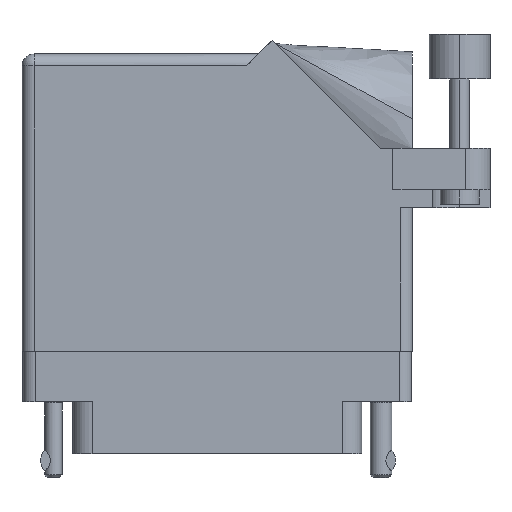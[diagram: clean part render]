
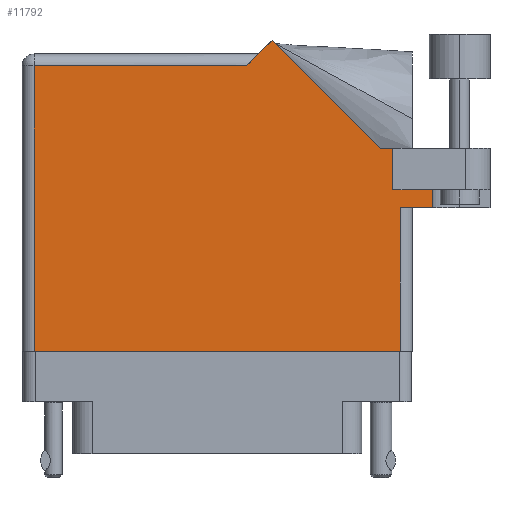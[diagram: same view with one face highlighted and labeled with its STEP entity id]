
A CAD part, front view. The second image highlights one B-rep face of the part: STEP entity #11792.
In plain terms, the highlighted face is planar.
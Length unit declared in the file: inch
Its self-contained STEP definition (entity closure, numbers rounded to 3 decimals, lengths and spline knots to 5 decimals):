
#990 = LINE ( 'NONE', #33582, #6879 ) ;
#1354 = ORIENTED_EDGE ( 'NONE', *, *, #5751, .T. ) ;
#2947 = CARTESIAN_POINT ( 'NONE',  ( 0., 1.53, 0. ) ) ;
#3234 = CARTESIAN_POINT ( 'NONE',  ( 1.91, 0.831, 0. ) ) ;
#4028 = CARTESIAN_POINT ( 'NONE',  ( 1.217, 1.53, 0. ) ) ;
#4146 = CARTESIAN_POINT ( 'NONE',  ( 0., 0., 0. ) ) ;
#4919 = CARTESIAN_POINT ( 'NONE',  ( 1.948, 0., 0. ) ) ;
#5751 = EDGE_CURVE ( 'NONE', #32708, #19872, #19036, .T. ) ;
#5757 = VECTOR ( 'NONE', #34159, 39.37008 ) ;
#6306 = LINE ( 'NONE', #43594, #44927 ) ;
#6641 = CARTESIAN_POINT ( 'NONE',  ( 1.91, 0.831, 0. ) ) ;
#6879 = VECTOR ( 'NONE', #7696, 39.37008 ) ;
#7042 = DIRECTION ( 'NONE',  ( -1., 0., 0. ) ) ;
#7444 = VECTOR ( 'NONE', #9508, 39.37008 ) ;
#7696 = DIRECTION ( 'NONE',  ( 0., -1., 0. ) ) ;
#8265 = FACE_OUTER_BOUND ( 'NONE', #32116, .T. ) ;
#8510 = LINE ( 'NONE', #40022, #17301 ) ;
#9508 = DIRECTION ( 'NONE',  ( -1., 0., 0. ) ) ;
#9732 = DIRECTION ( 'NONE',  ( 0., 1., 0. ) ) ;
#10441 = VERTEX_POINT ( 'NONE', #39763 ) ;
#10484 = EDGE_CURVE ( 'NONE', #25265, #26526, #45860, .T. ) ;
#10530 = CARTESIAN_POINT ( 'NONE',  ( 1.84442, 1.044, 0. ) ) ;
#11084 = ORIENTED_EDGE ( 'NONE', *, *, #30466, .T. ) ;
#11167 = VERTEX_POINT ( 'NONE', #33609 ) ;
#11792 = ADVANCED_FACE ( 'NONE', ( #8265 ), #36676, .F. ) ;
#12435 = VECTOR ( 'NONE', #26130, 39.37008 ) ;
#13024 = EDGE_CURVE ( 'NONE', #11167, #14028, #32784, .T. ) ;
#13460 = CARTESIAN_POINT ( 'NONE',  ( 1.948, 0.737, 0. ) ) ;
#13590 = ORIENTED_EDGE ( 'NONE', *, *, #48249, .T. ) ;
#13799 = VECTOR ( 'NONE', #9732, 39.37008 ) ;
#14028 = VERTEX_POINT ( 'NONE', #37925 ) ;
#14407 = EDGE_CURVE ( 'NONE', #19872, #45333, #6306, .T. ) ;
#14605 = EDGE_CURVE ( 'NONE', #26526, #11167, #41418, .T. ) ;
#16339 = VECTOR ( 'NONE', #47357, 39.37008 ) ;
#17117 = CARTESIAN_POINT ( 'NONE',  ( 2.1115, 0.831, 0. ) ) ;
#17301 = VECTOR ( 'NONE', #39360, 39.37008 ) ;
#18623 = LINE ( 'NONE', #4028, #5757 ) ;
#18814 = ORIENTED_EDGE ( 'NONE', *, *, #29938, .T. ) ;
#19036 = LINE ( 'NONE', #13460, #13799 ) ;
#19609 = CARTESIAN_POINT ( 'NONE',  ( 2.1115, 0.737, 0. ) ) ;
#19872 = VERTEX_POINT ( 'NONE', #42910 ) ;
#20058 = VERTEX_POINT ( 'NONE', #43712 ) ;
#20728 = ORIENTED_EDGE ( 'NONE', *, *, #45939, .F. ) ;
#21000 = ORIENTED_EDGE ( 'NONE', *, *, #13024, .T. ) ;
#21211 = DIRECTION ( 'NONE',  ( 1., 0., 0. ) ) ;
#23358 = ORIENTED_EDGE ( 'NONE', *, *, #14605, .T. ) ;
#25265 = VERTEX_POINT ( 'NONE', #6641 ) ;
#25728 = DIRECTION ( 'NONE',  ( 0., 0., -1. ) ) ;
#26130 = DIRECTION ( 'NONE',  ( 1., 0., 0. ) ) ;
#26526 = VERTEX_POINT ( 'NONE', #42178 ) ;
#26621 = LINE ( 'NONE', #32329, #41251 ) ;
#27088 = EDGE_CURVE ( 'NONE', #41062, #32708, #33568, .T. ) ;
#27171 = ORIENTED_EDGE ( 'NONE', *, *, #10484, .T. ) ;
#28191 = ORIENTED_EDGE ( 'NONE', *, *, #32321, .F. ) ;
#28197 = CARTESIAN_POINT ( 'NONE',  ( 0., 1.468, 0. ) ) ;
#29938 = EDGE_CURVE ( 'NONE', #14028, #10441, #18623, .T. ) ;
#30110 = CARTESIAN_POINT ( 'NONE',  ( 0.062, 0., 0. ) ) ;
#30195 = CARTESIAN_POINT ( 'NONE',  ( 2.41, 1.044, 0. ) ) ;
#30466 = EDGE_CURVE ( 'NONE', #10441, #20058, #34420, .T. ) ;
#30688 = DIRECTION ( 'NONE',  ( -1., 0., 0. ) ) ;
#32116 = EDGE_LOOP ( 'NONE', ( #41362, #1354, #46686, #20728, #28191, #27171, #23358, #21000, #18814, #11084, #13590 ) ) ;
#32321 = EDGE_CURVE ( 'NONE', #25265, #33697, #8510, .T. ) ;
#32329 = CARTESIAN_POINT ( 'NONE',  ( 0.062, 0., 0. ) ) ;
#32708 = VERTEX_POINT ( 'NONE', #4919 ) ;
#32784 = LINE ( 'NONE', #10530, #16339 ) ;
#33568 = LINE ( 'NONE', #4146, #12435 ) ;
#33582 = CARTESIAN_POINT ( 'NONE',  ( 2.1115, 1.16177, 0. ) ) ;
#33609 = CARTESIAN_POINT ( 'NONE',  ( 1.84442, 1.044, 0. ) ) ;
#33697 = VERTEX_POINT ( 'NONE', #17117 ) ;
#34159 = DIRECTION ( 'NONE',  ( -0.707, -0.707, 0. ) ) ;
#34420 = LINE ( 'NONE', #28197, #7444 ) ;
#35593 = DIRECTION ( 'NONE',  ( 0., -1., 0. ) ) ;
#35955 = VECTOR ( 'NONE', #37109, 39.37008 ) ;
#36676 = PLANE ( 'NONE',  #38304 ) ;
#37109 = DIRECTION ( 'NONE',  ( 0., 1., 0. ) ) ;
#37925 = CARTESIAN_POINT ( 'NONE',  ( 1.28771, 1.60071, 0. ) ) ;
#38304 = AXIS2_PLACEMENT_3D ( 'NONE', #2947, #25728, #7042 ) ;
#39360 = DIRECTION ( 'NONE',  ( 1., 0., 0. ) ) ;
#39763 = CARTESIAN_POINT ( 'NONE',  ( 1.155, 1.468, 0. ) ) ;
#40022 = CARTESIAN_POINT ( 'NONE',  ( 1.91, 0.831, 0. ) ) ;
#41062 = VERTEX_POINT ( 'NONE', #30110 ) ;
#41251 = VECTOR ( 'NONE', #35593, 39.37008 ) ;
#41362 = ORIENTED_EDGE ( 'NONE', *, *, #27088, .T. ) ;
#41418 = LINE ( 'NONE', #30195, #43733 ) ;
#42178 = CARTESIAN_POINT ( 'NONE',  ( 1.91, 1.044, 0. ) ) ;
#42910 = CARTESIAN_POINT ( 'NONE',  ( 1.948, 0.737, 0. ) ) ;
#43594 = CARTESIAN_POINT ( 'NONE',  ( 2.01, 0.737, 0. ) ) ;
#43712 = CARTESIAN_POINT ( 'NONE',  ( 0.062, 1.468, 0. ) ) ;
#43733 = VECTOR ( 'NONE', #30688, 39.37008 ) ;
#44927 = VECTOR ( 'NONE', #21211, 39.37008 ) ;
#45333 = VERTEX_POINT ( 'NONE', #19609 ) ;
#45860 = LINE ( 'NONE', #3234, #35955 ) ;
#45939 = EDGE_CURVE ( 'NONE', #33697, #45333, #990, .T. ) ;
#46686 = ORIENTED_EDGE ( 'NONE', *, *, #14407, .T. ) ;
#47357 = DIRECTION ( 'NONE',  ( -0.707, 0.707, 0. ) ) ;
#48249 = EDGE_CURVE ( 'NONE', #20058, #41062, #26621, .T. ) ;
